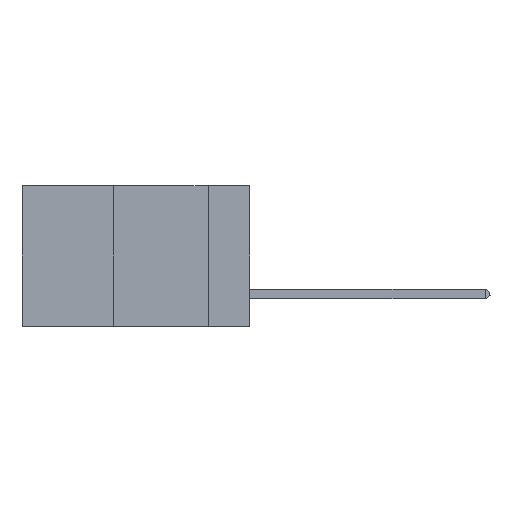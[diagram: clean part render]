
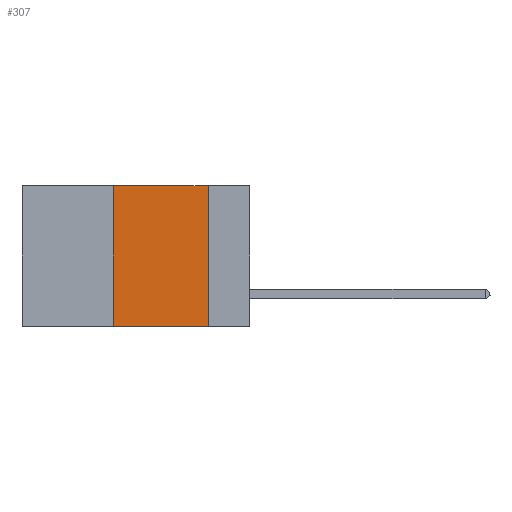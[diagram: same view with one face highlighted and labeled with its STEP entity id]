
A CAD part, left-side view. The second image highlights one B-rep face of the part: STEP entity #307.
In plain terms, the highlighted planar face has unit normal (-1, 0, 0).
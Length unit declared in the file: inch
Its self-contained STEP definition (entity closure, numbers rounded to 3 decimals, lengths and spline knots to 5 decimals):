
#307 = ADVANCED_FACE ( 'NONE', ( #9076 ), #3705, .F. ) ;
#542 = CARTESIAN_POINT ( 'NONE',  ( 0., 0.6, -0.37 ) ) ;
#1194 = AXIS2_PLACEMENT_3D ( 'NONE', #9164, #2808, #4466 ) ;
#1287 = EDGE_CURVE ( 'NONE', #5365, #3751, #8212, .T. ) ;
#1332 = DIRECTION ( 'NONE',  ( 0., -1., 0. ) ) ;
#1688 = CARTESIAN_POINT ( 'NONE',  ( 0., 0.36, 0. ) ) ;
#2198 = DIRECTION ( 'NONE',  ( 0., 0., -1. ) ) ;
#2510 = EDGE_CURVE ( 'NONE', #3743, #5365, #6891, .T. ) ;
#2808 = DIRECTION ( 'NONE',  ( 1., 0., 0. ) ) ;
#3568 = ORIENTED_EDGE ( 'NONE', *, *, #10059, .T. ) ;
#3693 = VECTOR ( 'NONE', #8216, 39.37008 ) ;
#3705 = PLANE ( 'NONE',  #1194 ) ;
#3743 = VERTEX_POINT ( 'NONE', #1688 ) ;
#3751 = VERTEX_POINT ( 'NONE', #5682 ) ;
#4262 = ORIENTED_EDGE ( 'NONE', *, *, #9387, .F. ) ;
#4466 = DIRECTION ( 'NONE',  ( 0., 0., -1. ) ) ;
#5193 = ORIENTED_EDGE ( 'NONE', *, *, #1287, .F. ) ;
#5336 = CARTESIAN_POINT ( 'NONE',  ( 0., 0.11, 0. ) ) ;
#5365 = VERTEX_POINT ( 'NONE', #5336 ) ;
#5368 = VECTOR ( 'NONE', #2198, 39.37008 ) ;
#5682 = CARTESIAN_POINT ( 'NONE',  ( 0., 0.11, -0.37 ) ) ;
#6272 = EDGE_LOOP ( 'NONE', ( #5193, #9258, #4262, #3568 ) ) ;
#6497 = CARTESIAN_POINT ( 'NONE',  ( 0., 0.6, 0. ) ) ;
#6672 = DIRECTION ( 'NONE',  ( 0., -1., 0. ) ) ;
#6891 = LINE ( 'NONE', #6497, #7636 ) ;
#7636 = VECTOR ( 'NONE', #6672, 39.37008 ) ;
#8056 = LINE ( 'NONE', #542, #9066 ) ;
#8212 = LINE ( 'NONE', #9219, #5368 ) ;
#8216 = DIRECTION ( 'NONE',  ( 0., 0., 1. ) ) ;
#9066 = VECTOR ( 'NONE', #1332, 39.37008 ) ;
#9076 = FACE_OUTER_BOUND ( 'NONE', #6272, .T. ) ;
#9164 = CARTESIAN_POINT ( 'NONE',  ( 0., 0.6, 0. ) ) ;
#9206 = VERTEX_POINT ( 'NONE', #9431 ) ;
#9219 = CARTESIAN_POINT ( 'NONE',  ( 0., 0.11, 0. ) ) ;
#9258 = ORIENTED_EDGE ( 'NONE', *, *, #2510, .F. ) ;
#9387 = EDGE_CURVE ( 'NONE', #9206, #3743, #9801, .T. ) ;
#9431 = CARTESIAN_POINT ( 'NONE',  ( 0., 0.36, -0.37 ) ) ;
#9715 = CARTESIAN_POINT ( 'NONE',  ( 0., 0.36, 0. ) ) ;
#9801 = LINE ( 'NONE', #9715, #3693 ) ;
#10059 = EDGE_CURVE ( 'NONE', #9206, #3751, #8056, .T. ) ;
